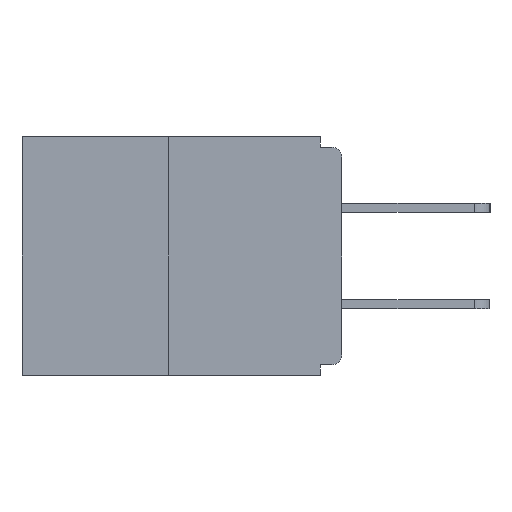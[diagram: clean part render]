
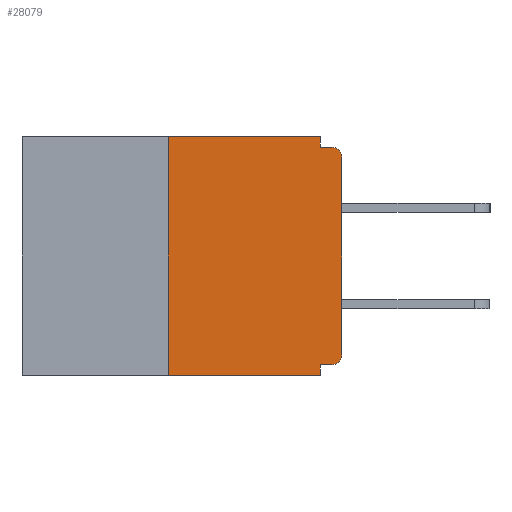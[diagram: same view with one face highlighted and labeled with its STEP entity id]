
A CAD part, left-side view. The second image highlights one B-rep face of the part: STEP entity #28079.
In plain terms, the highlighted planar face has unit normal (-1, 0, 0).
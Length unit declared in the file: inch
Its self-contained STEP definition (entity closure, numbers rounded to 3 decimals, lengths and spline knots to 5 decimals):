
#593 = AXIS2_PLACEMENT_3D ( 'NONE', #24089, #17125, #12784 ) ;
#850 = VECTOR ( 'NONE', #2435, 39.37008 ) ;
#2025 = VECTOR ( 'NONE', #7722, 39.37008 ) ;
#2200 = AXIS2_PLACEMENT_3D ( 'NONE', #17150, #3002, #5789 ) ;
#2430 = ORIENTED_EDGE ( 'NONE', *, *, #5977, .T. ) ;
#2435 = DIRECTION ( 'NONE',  ( 0., 0., -1. ) ) ;
#2581 = LINE ( 'NONE', #16595, #850 ) ;
#2849 = VERTEX_POINT ( 'NONE', #5427 ) ;
#2973 = CIRCLE ( 'NONE', #593, 0.015 ) ;
#3002 = DIRECTION ( 'NONE',  ( 1., 0., 0. ) ) ;
#3367 = LINE ( 'NONE', #12726, #22482 ) ;
#3444 = CIRCLE ( 'NONE', #8645, 0.015 ) ;
#4011 = ORIENTED_EDGE ( 'NONE', *, *, #19254, .F. ) ;
#4650 = CARTESIAN_POINT ( 'NONE',  ( 0., 0., 0. ) ) ;
#4785 = VERTEX_POINT ( 'NONE', #22562 ) ;
#5427 = CARTESIAN_POINT ( 'NONE',  ( 0., 0.031, 0. ) ) ;
#5507 = FACE_OUTER_BOUND ( 'NONE', #14122, .T. ) ;
#5789 = DIRECTION ( 'NONE',  ( 0., 0., -1. ) ) ;
#5977 = EDGE_CURVE ( 'NONE', #25875, #13751, #3367, .T. ) ;
#6049 = CARTESIAN_POINT ( 'NONE',  ( 0., 0.25, 0. ) ) ;
#6412 = VECTOR ( 'NONE', #22615, 39.37008 ) ;
#6506 = CARTESIAN_POINT ( 'NONE',  ( 0., 0.25, -0.343 ) ) ;
#6527 = EDGE_CURVE ( 'NONE', #4785, #27362, #3444, .T. ) ;
#7230 = EDGE_CURVE ( 'NONE', #2849, #21206, #26348, .T. ) ;
#7358 = DIRECTION ( 'NONE',  ( 0., -1., 0. ) ) ;
#7719 = CARTESIAN_POINT ( 'NONE',  ( 0., 0.015, -0.015 ) ) ;
#7722 = DIRECTION ( 'NONE',  ( 0., 0., -1. ) ) ;
#8249 = EDGE_CURVE ( 'NONE', #15210, #16321, #2973, .T. ) ;
#8645 = AXIS2_PLACEMENT_3D ( 'NONE', #15687, #24768, #29363 ) ;
#8953 = LINE ( 'NONE', #4650, #17043 ) ;
#9065 = ORIENTED_EDGE ( 'NONE', *, *, #9572, .T. ) ;
#9572 = EDGE_CURVE ( 'NONE', #16321, #4785, #8953, .T. ) ;
#9658 = CARTESIAN_POINT ( 'NONE',  ( 0., 0.25, 0. ) ) ;
#10867 = CARTESIAN_POINT ( 'NONE',  ( 0., 0.015, -0.328 ) ) ;
#10905 = ORIENTED_EDGE ( 'NONE', *, *, #28970, .F. ) ;
#12278 = VERTEX_POINT ( 'NONE', #17401 ) ;
#12726 = CARTESIAN_POINT ( 'NONE',  ( 0., 0.46, -0.343 ) ) ;
#12784 = DIRECTION ( 'NONE',  ( 0., 0., -1. ) ) ;
#13077 = DIRECTION ( 'NONE',  ( 0., 0., 1. ) ) ;
#13087 = CARTESIAN_POINT ( 'NONE',  ( 0., 0., -0.328 ) ) ;
#13699 = ORIENTED_EDGE ( 'NONE', *, *, #27121, .F. ) ;
#13751 = VERTEX_POINT ( 'NONE', #21050 ) ;
#13752 = DIRECTION ( 'NONE',  ( 0., 0., 1. ) ) ;
#14122 = EDGE_LOOP ( 'NONE', ( #10905, #4011, #2430, #15132, #13699, #29425, #9065, #18763, #28875, #27675 ) ) ;
#14533 = CARTESIAN_POINT ( 'NONE',  ( 0., 0.46, 0. ) ) ;
#15132 = ORIENTED_EDGE ( 'NONE', *, *, #23970, .F. ) ;
#15210 = VERTEX_POINT ( 'NONE', #10867 ) ;
#15687 = CARTESIAN_POINT ( 'NONE',  ( 0., 0.015, -0.03 ) ) ;
#15760 = VECTOR ( 'NONE', #13077, 39.37008 ) ;
#16321 = VERTEX_POINT ( 'NONE', #26005 ) ;
#16595 = CARTESIAN_POINT ( 'NONE',  ( 0., 0.031, -0.343 ) ) ;
#17043 = VECTOR ( 'NONE', #13752, 39.37008 ) ;
#17125 = DIRECTION ( 'NONE',  ( -1., 0., 0. ) ) ;
#17150 = CARTESIAN_POINT ( 'NONE',  ( 0., 0.46, 0. ) ) ;
#17401 = CARTESIAN_POINT ( 'NONE',  ( 0., 0.031, -0.328 ) ) ;
#17835 = CARTESIAN_POINT ( 'NONE',  ( 0., 0., -0.015 ) ) ;
#17960 = VECTOR ( 'NONE', #7358, 39.37008 ) ;
#18763 = ORIENTED_EDGE ( 'NONE', *, *, #6527, .T. ) ;
#19254 = EDGE_CURVE ( 'NONE', #25875, #20755, #24096, .T. ) ;
#19332 = VECTOR ( 'NONE', #24401, 39.37008 ) ;
#20594 = EDGE_CURVE ( 'NONE', #21206, #27362, #27099, .T. ) ;
#20755 = VERTEX_POINT ( 'NONE', #9658 ) ;
#21050 = CARTESIAN_POINT ( 'NONE',  ( 0., 0.031, -0.343 ) ) ;
#21206 = VERTEX_POINT ( 'NONE', #26405 ) ;
#21801 = DIRECTION ( 'NONE',  ( 0., -1., 0. ) ) ;
#22482 = VECTOR ( 'NONE', #21801, 39.37008 ) ;
#22562 = CARTESIAN_POINT ( 'NONE',  ( 0., 0., -0.03 ) ) ;
#22615 = DIRECTION ( 'NONE',  ( 0., 1., 0. ) ) ;
#23311 = LINE ( 'NONE', #14533, #17960 ) ;
#23970 = EDGE_CURVE ( 'NONE', #12278, #13751, #2581, .T. ) ;
#24089 = CARTESIAN_POINT ( 'NONE',  ( 0., 0.015, -0.313 ) ) ;
#24096 = LINE ( 'NONE', #6049, #15760 ) ;
#24401 = DIRECTION ( 'NONE',  ( 0., -1., 0. ) ) ;
#24559 = LINE ( 'NONE', #13087, #6412 ) ;
#24768 = DIRECTION ( 'NONE',  ( -1., 0., 0. ) ) ;
#25810 = PLANE ( 'NONE',  #2200 ) ;
#25875 = VERTEX_POINT ( 'NONE', #6506 ) ;
#26005 = CARTESIAN_POINT ( 'NONE',  ( 0., 0., -0.313 ) ) ;
#26210 = CARTESIAN_POINT ( 'NONE',  ( 0., 0.031, 0. ) ) ;
#26348 = LINE ( 'NONE', #26210, #2025 ) ;
#26405 = CARTESIAN_POINT ( 'NONE',  ( 0., 0.031, -0.015 ) ) ;
#27099 = LINE ( 'NONE', #17835, #19332 ) ;
#27121 = EDGE_CURVE ( 'NONE', #15210, #12278, #24559, .T. ) ;
#27362 = VERTEX_POINT ( 'NONE', #7719 ) ;
#27675 = ORIENTED_EDGE ( 'NONE', *, *, #7230, .F. ) ;
#28079 = ADVANCED_FACE ( 'NONE', ( #5507 ), #25810, .F. ) ;
#28875 = ORIENTED_EDGE ( 'NONE', *, *, #20594, .F. ) ;
#28970 = EDGE_CURVE ( 'NONE', #20755, #2849, #23311, .T. ) ;
#29363 = DIRECTION ( 'NONE',  ( 0., 0., -1. ) ) ;
#29425 = ORIENTED_EDGE ( 'NONE', *, *, #8249, .T. ) ;
